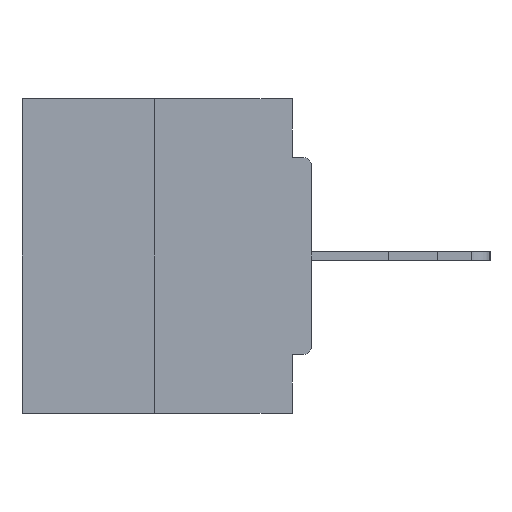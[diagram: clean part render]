
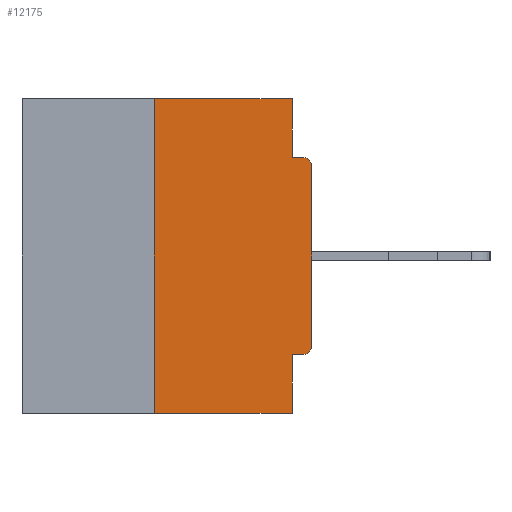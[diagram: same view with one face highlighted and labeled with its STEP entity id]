
A CAD part, left-side view. The second image highlights one B-rep face of the part: STEP entity #12175.
In plain terms, the highlighted planar face has unit normal (-1, 0, 0).
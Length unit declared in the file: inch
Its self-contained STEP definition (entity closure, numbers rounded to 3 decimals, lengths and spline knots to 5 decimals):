
#146 = EDGE_CURVE ( 'NONE', #37195, #7449, #34006, .T. ) ;
#465 = DIRECTION ( 'NONE',  ( 0., 0., 1. ) ) ;
#573 = DIRECTION ( 'NONE',  ( 0., 0., -1. ) ) ;
#681 = AXIS2_PLACEMENT_3D ( 'NONE', #13995, #19789, #37179 ) ;
#689 = VERTEX_POINT ( 'NONE', #991 ) ;
#991 = CARTESIAN_POINT ( 'NONE',  ( 0., 0.25, -0.5 ) ) ;
#1552 = CARTESIAN_POINT ( 'NONE',  ( 0., 0., -0.4065 ) ) ;
#1684 = DIRECTION ( 'NONE',  ( 0., 0., -1. ) ) ;
#2116 = EDGE_CURVE ( 'NONE', #36538, #10992, #35879, .T. ) ;
#2171 = ORIENTED_EDGE ( 'NONE', *, *, #17765, .F. ) ;
#2600 = CARTESIAN_POINT ( 'NONE',  ( 0., 0., -0.3915 ) ) ;
#3171 = ORIENTED_EDGE ( 'NONE', *, *, #2116, .F. ) ;
#3720 = DIRECTION ( 'NONE',  ( 0., 0., 1. ) ) ;
#3814 = ORIENTED_EDGE ( 'NONE', *, *, #12143, .F. ) ;
#3956 = CARTESIAN_POINT ( 'NONE',  ( 0., 0.25, 0. ) ) ;
#4304 = CARTESIAN_POINT ( 'NONE',  ( 0., 0., -0.0935 ) ) ;
#4652 = EDGE_CURVE ( 'NONE', #27531, #23380, #6561, .T. ) ;
#6296 = ORIENTED_EDGE ( 'NONE', *, *, #26223, .F. ) ;
#6561 = LINE ( 'NONE', #33186, #24653 ) ;
#7449 = VERTEX_POINT ( 'NONE', #36102 ) ;
#7479 = CARTESIAN_POINT ( 'NONE',  ( 0., 0.015, -0.3915 ) ) ;
#8600 = VECTOR ( 'NONE', #465, 39.37008 ) ;
#8649 = CARTESIAN_POINT ( 'NONE',  ( 0., 0.031, -0.0935 ) ) ;
#10966 = DIRECTION ( 'NONE',  ( 0., -1., 0. ) ) ;
#10992 = VERTEX_POINT ( 'NONE', #22373 ) ;
#11163 = EDGE_LOOP ( 'NONE', ( #28324, #2171, #24318, #3171, #6296, #26933, #19703, #19424, #3814, #13608 ) ) ;
#11346 = EDGE_CURVE ( 'NONE', #25032, #38145, #30117, .T. ) ;
#12143 = EDGE_CURVE ( 'NONE', #24701, #7449, #24926, .T. ) ;
#12175 = ADVANCED_FACE ( 'NONE', ( #12906 ), #18105, .F. ) ;
#12906 = FACE_OUTER_BOUND ( 'NONE', #11163, .T. ) ;
#13608 = ORIENTED_EDGE ( 'NONE', *, *, #16322, .F. ) ;
#13995 = CARTESIAN_POINT ( 'NONE',  ( 0., 0.015, -0.1085 ) ) ;
#14238 = CARTESIAN_POINT ( 'NONE',  ( 0., 0.031, 0. ) ) ;
#16051 = DIRECTION ( 'NONE',  ( 0., -1., 0. ) ) ;
#16195 = LINE ( 'NONE', #1552, #33088 ) ;
#16322 = EDGE_CURVE ( 'NONE', #23380, #24701, #34300, .T. ) ;
#16410 = VECTOR ( 'NONE', #3720, 39.37008 ) ;
#17765 = EDGE_CURVE ( 'NONE', #689, #27531, #27666, .T. ) ;
#18105 = PLANE ( 'NONE',  #23993 ) ;
#18494 = DIRECTION ( 'NONE',  ( 0., -1., 0. ) ) ;
#18683 = VECTOR ( 'NONE', #1684, 39.37008 ) ;
#19131 = LINE ( 'NONE', #24340, #16410 ) ;
#19221 = DIRECTION ( 'NONE',  ( -1., 0., 0. ) ) ;
#19424 = ORIENTED_EDGE ( 'NONE', *, *, #146, .T. ) ;
#19703 = ORIENTED_EDGE ( 'NONE', *, *, #29112, .T. ) ;
#19789 = DIRECTION ( 'NONE',  ( -1., 0., 0. ) ) ;
#20710 = CARTESIAN_POINT ( 'NONE',  ( 0., 0.031, -0.4065 ) ) ;
#21040 = VECTOR ( 'NONE', #10966, 39.37008 ) ;
#21593 = VECTOR ( 'NONE', #36249, 39.37008 ) ;
#22047 = EDGE_CURVE ( 'NONE', #689, #10992, #25438, .T. ) ;
#22373 = CARTESIAN_POINT ( 'NONE',  ( 0., 0.031, -0.5 ) ) ;
#23380 = VERTEX_POINT ( 'NONE', #14238 ) ;
#23636 = CARTESIAN_POINT ( 'NONE',  ( 0., 0.015, -0.4065 ) ) ;
#23993 = AXIS2_PLACEMENT_3D ( 'NONE', #36270, #35892, #573 ) ;
#24318 = ORIENTED_EDGE ( 'NONE', *, *, #22047, .T. ) ;
#24340 = CARTESIAN_POINT ( 'NONE',  ( 0., 0., 0. ) ) ;
#24653 = VECTOR ( 'NONE', #18494, 39.37008 ) ;
#24701 = VERTEX_POINT ( 'NONE', #8649 ) ;
#24926 = LINE ( 'NONE', #4304, #35123 ) ;
#25032 = VERTEX_POINT ( 'NONE', #23636 ) ;
#25438 = LINE ( 'NONE', #31621, #21040 ) ;
#26223 = EDGE_CURVE ( 'NONE', #25032, #36538, #16195, .T. ) ;
#26933 = ORIENTED_EDGE ( 'NONE', *, *, #11346, .T. ) ;
#27531 = VERTEX_POINT ( 'NONE', #31471 ) ;
#27666 = LINE ( 'NONE', #3956, #8600 ) ;
#28324 = ORIENTED_EDGE ( 'NONE', *, *, #4652, .F. ) ;
#29112 = EDGE_CURVE ( 'NONE', #38145, #37195, #19131, .T. ) ;
#30117 = CIRCLE ( 'NONE', #33210, 0.015 ) ;
#30298 = DIRECTION ( 'NONE',  ( 0., 1., 0. ) ) ;
#31014 = CARTESIAN_POINT ( 'NONE',  ( 0., 0.031, 0. ) ) ;
#31024 = DIRECTION ( 'NONE',  ( 0., 0., -1. ) ) ;
#31471 = CARTESIAN_POINT ( 'NONE',  ( 0., 0.25, 0. ) ) ;
#31621 = CARTESIAN_POINT ( 'NONE',  ( 0., 0.46, -0.5 ) ) ;
#32668 = CARTESIAN_POINT ( 'NONE',  ( 0., 0., -0.1085 ) ) ;
#32986 = CARTESIAN_POINT ( 'NONE',  ( 0., 0.031, -0.5 ) ) ;
#33088 = VECTOR ( 'NONE', #30298, 39.37008 ) ;
#33186 = CARTESIAN_POINT ( 'NONE',  ( 0., 0.46, 0. ) ) ;
#33210 = AXIS2_PLACEMENT_3D ( 'NONE', #7479, #19221, #31024 ) ;
#34006 = CIRCLE ( 'NONE', #681, 0.015 ) ;
#34300 = LINE ( 'NONE', #31014, #18683 ) ;
#35123 = VECTOR ( 'NONE', #16051, 39.37008 ) ;
#35879 = LINE ( 'NONE', #32986, #21593 ) ;
#35892 = DIRECTION ( 'NONE',  ( 1., 0., 0. ) ) ;
#36102 = CARTESIAN_POINT ( 'NONE',  ( 0., 0.015, -0.0935 ) ) ;
#36249 = DIRECTION ( 'NONE',  ( 0., 0., -1. ) ) ;
#36270 = CARTESIAN_POINT ( 'NONE',  ( 0., 0.46, 0. ) ) ;
#36538 = VERTEX_POINT ( 'NONE', #20710 ) ;
#37179 = DIRECTION ( 'NONE',  ( 0., 0., -1. ) ) ;
#37195 = VERTEX_POINT ( 'NONE', #32668 ) ;
#38145 = VERTEX_POINT ( 'NONE', #2600 ) ;
